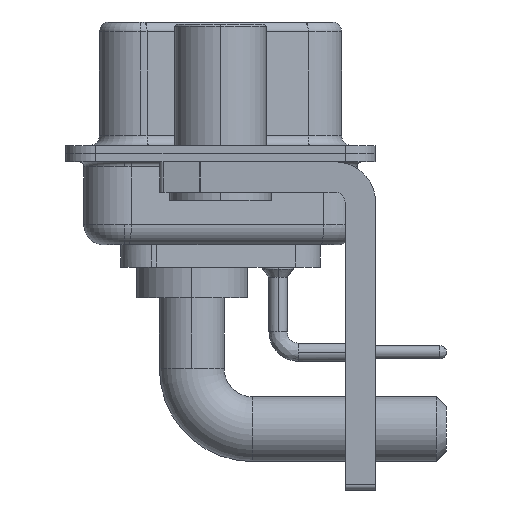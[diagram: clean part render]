
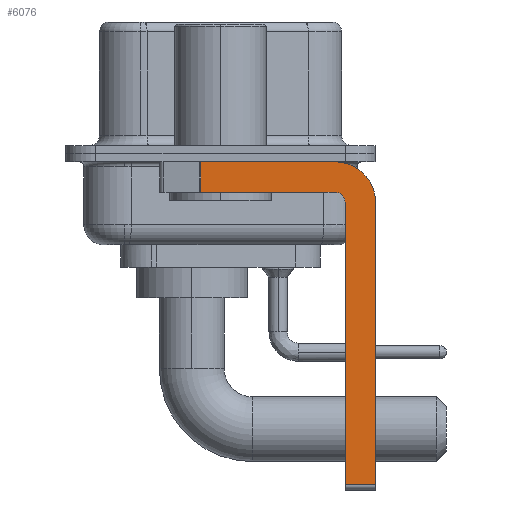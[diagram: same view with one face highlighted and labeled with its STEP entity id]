
A CAD part, left-side view. The second image highlights one B-rep face of the part: STEP entity #6076.
In plain terms, the highlighted planar face has unit normal (-1, 0, 0).
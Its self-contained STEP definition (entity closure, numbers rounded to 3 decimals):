
#815 = DIRECTION ( 'NONE',  ( 0., 0., -1. ) ) ;
#833 = VERTEX_POINT ( 'NONE', #15855 ) ;
#1209 = DIRECTION ( 'NONE',  ( 1., 0., 0. ) ) ;
#1277 = ORIENTED_EDGE ( 'NONE', *, *, #16813, .F. ) ;
#1497 = ORIENTED_EDGE ( 'NONE', *, *, #21938, .T. ) ;
#1716 = DIRECTION ( 'NONE',  ( -1., 0., 0. ) ) ;
#1724 = VERTEX_POINT ( 'NONE', #8453 ) ;
#2419 = LINE ( 'NONE', #18441, #15492 ) ;
#2689 = EDGE_CURVE ( 'NONE', #833, #15945, #13281, .T. ) ;
#3010 = CARTESIAN_POINT ( 'NONE',  ( -2.9, 0.978, -1.9 ) ) ;
#3213 = CARTESIAN_POINT ( 'NONE',  ( -2.9, -5.65, -0.4 ) ) ;
#3461 = EDGE_CURVE ( 'NONE', #833, #6861, #12835, .T. ) ;
#3942 = DIRECTION ( 'NONE',  ( 0., 0., -1. ) ) ;
#4195 = VERTEX_POINT ( 'NONE', #8229 ) ;
#5133 = LINE ( 'NONE', #11001, #13401 ) ;
#5666 = ORIENTED_EDGE ( 'NONE', *, *, #22093, .F. ) ;
#5728 = CARTESIAN_POINT ( 'NONE',  ( -2.9, -5.65, -2.4 ) ) ;
#5776 = AXIS2_PLACEMENT_3D ( 'NONE', #5728, #1716, #16745 ) ;
#6076 = ADVANCED_FACE ( 'NONE', ( #16091 ), #20345, .F. ) ;
#6361 = EDGE_CURVE ( 'NONE', #1724, #26319, #13783, .T. ) ;
#6376 = VECTOR ( 'NONE', #21396, 1000. ) ;
#6861 = VERTEX_POINT ( 'NONE', #3213 ) ;
#8229 = CARTESIAN_POINT ( 'NONE',  ( -2.9, -7.65, -16.35 ) ) ;
#8453 = CARTESIAN_POINT ( 'NONE',  ( -2.9, -6.15, -16.35 ) ) ;
#9009 = DIRECTION ( 'NONE',  ( 0., 1., 0. ) ) ;
#9209 = EDGE_LOOP ( 'NONE', ( #18198, #10775, #26128, #22604, #24407, #1497, #1277, #5666 ) ) ;
#10705 = DIRECTION ( 'NONE',  ( 0., -1., 0. ) ) ;
#10775 = ORIENTED_EDGE ( 'NONE', *, *, #2689, .T. ) ;
#11001 = CARTESIAN_POINT ( 'NONE',  ( -2.9, -5.65, -1.9 ) ) ;
#11223 = CARTESIAN_POINT ( 'NONE',  ( -2.9, 0.978, -1.9 ) ) ;
#12228 = VECTOR ( 'NONE', #21428, 1000. ) ;
#12835 = LINE ( 'NONE', #20716, #19486 ) ;
#13175 = AXIS2_PLACEMENT_3D ( 'NONE', #18334, #22221, #3942 ) ;
#13281 = LINE ( 'NONE', #3010, #12228 ) ;
#13359 = CARTESIAN_POINT ( 'NONE',  ( -2.9, -5.65, -2.4 ) ) ;
#13401 = VECTOR ( 'NONE', #9009, 1000. ) ;
#13428 = LINE ( 'NONE', #21577, #21651 ) ;
#13783 = LINE ( 'NONE', #21667, #6376 ) ;
#13917 = EDGE_CURVE ( 'NONE', #26319, #15539, #26235, .T. ) ;
#15492 = VECTOR ( 'NONE', #10705, 1000. ) ;
#15539 = VERTEX_POINT ( 'NONE', #15931 ) ;
#15855 = CARTESIAN_POINT ( 'NONE',  ( -2.9, 0.978, -0.4 ) ) ;
#15931 = CARTESIAN_POINT ( 'NONE',  ( -2.9, -5.65, -1.9 ) ) ;
#15945 = VERTEX_POINT ( 'NONE', #11223 ) ;
#16091 = FACE_OUTER_BOUND ( 'NONE', #9209, .T. ) ;
#16745 = DIRECTION ( 'NONE',  ( 0., 0., 1. ) ) ;
#16813 = EDGE_CURVE ( 'NONE', #22120, #4195, #13428, .T. ) ;
#16978 = DIRECTION ( 'NONE',  ( 0., -1., 0. ) ) ;
#18198 = ORIENTED_EDGE ( 'NONE', *, *, #3461, .F. ) ;
#18334 = CARTESIAN_POINT ( 'NONE',  ( -2.9, -5.65, -2.4 ) ) ;
#18441 = CARTESIAN_POINT ( 'NONE',  ( -2.9, -5.65, -16.35 ) ) ;
#19486 = VECTOR ( 'NONE', #16978, 1000. ) ;
#19768 = CIRCLE ( 'NONE', #24427, 2. ) ;
#20345 = PLANE ( 'NONE',  #13175 ) ;
#20716 = CARTESIAN_POINT ( 'NONE',  ( -2.9, 3., -0.4 ) ) ;
#21396 = DIRECTION ( 'NONE',  ( 0., 0., 1. ) ) ;
#21428 = DIRECTION ( 'NONE',  ( 0., 0., -1. ) ) ;
#21577 = CARTESIAN_POINT ( 'NONE',  ( -2.9, -7.65, -2.4 ) ) ;
#21651 = VECTOR ( 'NONE', #25445, 1000. ) ;
#21667 = CARTESIAN_POINT ( 'NONE',  ( -2.9, -6.15, -16.6 ) ) ;
#21938 = EDGE_CURVE ( 'NONE', #1724, #4195, #2419, .T. ) ;
#22093 = EDGE_CURVE ( 'NONE', #6861, #22120, #19768, .T. ) ;
#22120 = VERTEX_POINT ( 'NONE', #22163 ) ;
#22163 = CARTESIAN_POINT ( 'NONE',  ( -2.9, -7.65, -2.4 ) ) ;
#22221 = DIRECTION ( 'NONE',  ( 1., 0., 0. ) ) ;
#22604 = ORIENTED_EDGE ( 'NONE', *, *, #13917, .F. ) ;
#23035 = EDGE_CURVE ( 'NONE', #15539, #15945, #5133, .T. ) ;
#24131 = CARTESIAN_POINT ( 'NONE',  ( -2.9, -6.15, -2.4 ) ) ;
#24407 = ORIENTED_EDGE ( 'NONE', *, *, #6361, .F. ) ;
#24427 = AXIS2_PLACEMENT_3D ( 'NONE', #13359, #1209, #815 ) ;
#25445 = DIRECTION ( 'NONE',  ( 0., 0., -1. ) ) ;
#26128 = ORIENTED_EDGE ( 'NONE', *, *, #23035, .F. ) ;
#26235 = CIRCLE ( 'NONE', #5776, 0.5 ) ;
#26319 = VERTEX_POINT ( 'NONE', #24131 ) ;
